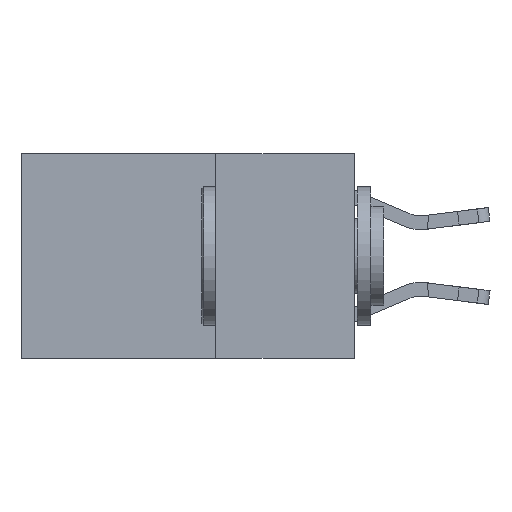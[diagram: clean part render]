
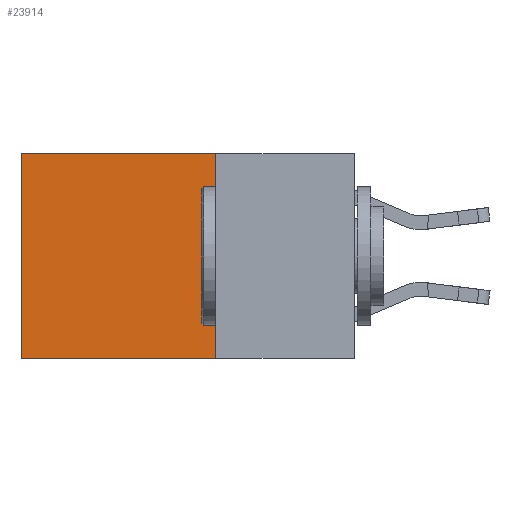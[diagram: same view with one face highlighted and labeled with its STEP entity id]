
A CAD part, left-side view. The second image highlights one B-rep face of the part: STEP entity #23914.
In plain terms, the highlighted planar face has unit normal (-1, 0, 0).
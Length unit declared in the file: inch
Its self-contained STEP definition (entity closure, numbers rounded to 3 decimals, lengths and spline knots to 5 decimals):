
#1591 = ORIENTED_EDGE ( 'NONE', *, *, #18653, .T. ) ;
#3366 = CARTESIAN_POINT ( 'NONE',  ( 0.2625, 0.25, -0.37 ) ) ;
#3461 = VERTEX_POINT ( 'NONE', #18925 ) ;
#3562 = CARTESIAN_POINT ( 'NONE',  ( 0.2625, 0.25, 0. ) ) ;
#4726 = VERTEX_POINT ( 'NONE', #14683 ) ;
#5127 = DIRECTION ( 'NONE',  ( 0., 0., -1. ) ) ;
#5835 = DIRECTION ( 'NONE',  ( 0., 0., -1. ) ) ;
#8900 = ORIENTED_EDGE ( 'NONE', *, *, #20370, .T. ) ;
#11546 = CARTESIAN_POINT ( 'NONE',  ( 0.2625, 0.25, -0.37 ) ) ;
#12170 = LINE ( 'NONE', #18470, #23283 ) ;
#12235 = FACE_OUTER_BOUND ( 'NONE', #24758, .T. ) ;
#12685 = EDGE_CURVE ( 'NONE', #4726, #20092, #24787, .T. ) ;
#13214 = CARTESIAN_POINT ( 'NONE',  ( 0.2625, 0.6, 0. ) ) ;
#14473 = VECTOR ( 'NONE', #28011, 39.37008 ) ;
#14665 = ORIENTED_EDGE ( 'NONE', *, *, #12685, .F. ) ;
#14683 = CARTESIAN_POINT ( 'NONE',  ( 0.2625, 0.25, 0. ) ) ;
#15163 = LINE ( 'NONE', #25768, #14473 ) ;
#17208 = VECTOR ( 'NONE', #27111, 39.37008 ) ;
#18470 = CARTESIAN_POINT ( 'NONE',  ( 0.2625, 0.6, 0. ) ) ;
#18653 = EDGE_CURVE ( 'NONE', #22670, #3461, #12170, .T. ) ;
#18925 = CARTESIAN_POINT ( 'NONE',  ( 0.2625, 0.6, -0.37 ) ) ;
#19174 = DIRECTION ( 'NONE',  ( 1., 0., 0. ) ) ;
#20092 = VERTEX_POINT ( 'NONE', #3366 ) ;
#20370 = EDGE_CURVE ( 'NONE', #4726, #22670, #15163, .T. ) ;
#20752 = EDGE_CURVE ( 'NONE', #20092, #3461, #22444, .T. ) ;
#22142 = DIRECTION ( 'NONE',  ( 0., 0., -1. ) ) ;
#22444 = LINE ( 'NONE', #11546, #17208 ) ;
#22670 = VERTEX_POINT ( 'NONE', #13214 ) ;
#23283 = VECTOR ( 'NONE', #5127, 39.37008 ) ;
#23914 = ADVANCED_FACE ( 'NONE', ( #12235 ), #28071, .F. ) ;
#24081 = VECTOR ( 'NONE', #22142, 39.37008 ) ;
#24395 = CARTESIAN_POINT ( 'NONE',  ( 0.2625, 0.25, 0. ) ) ;
#24741 = AXIS2_PLACEMENT_3D ( 'NONE', #3562, #19174, #5835 ) ;
#24758 = EDGE_LOOP ( 'NONE', ( #1591, #26046, #14665, #8900 ) ) ;
#24787 = LINE ( 'NONE', #24395, #24081 ) ;
#25768 = CARTESIAN_POINT ( 'NONE',  ( 0.2625, 0.25, 0. ) ) ;
#26046 = ORIENTED_EDGE ( 'NONE', *, *, #20752, .F. ) ;
#27111 = DIRECTION ( 'NONE',  ( 0., 1., 0. ) ) ;
#28011 = DIRECTION ( 'NONE',  ( 0., 1., 0. ) ) ;
#28071 = PLANE ( 'NONE',  #24741 ) ;
